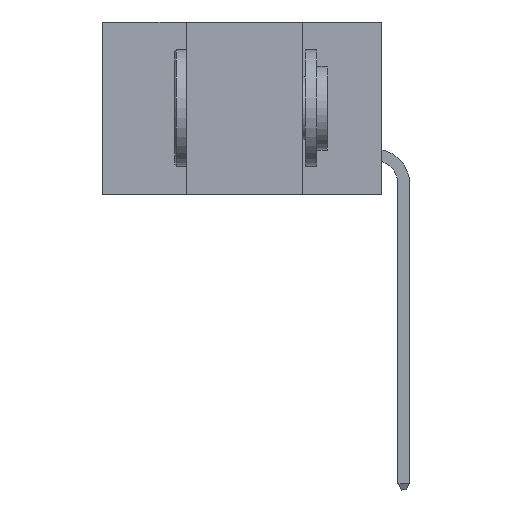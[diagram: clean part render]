
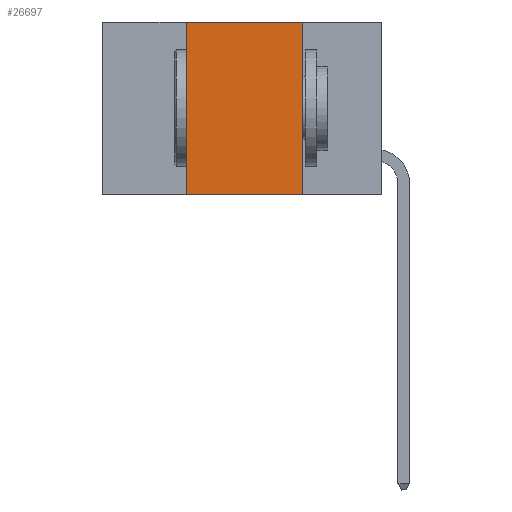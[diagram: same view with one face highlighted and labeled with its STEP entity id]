
A CAD part, left-side view. The second image highlights one B-rep face of the part: STEP entity #26697.
In plain terms, the highlighted planar face has unit normal (-1, 0, 0).
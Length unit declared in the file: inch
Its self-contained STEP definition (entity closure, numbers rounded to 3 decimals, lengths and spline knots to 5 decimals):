
#749 = ORIENTED_EDGE ( 'NONE', *, *, #1945, .F. ) ;
#993 = VERTEX_POINT ( 'NONE', #15844 ) ;
#1127 = CARTESIAN_POINT ( 'NONE',  ( 0., 0.17, 0. ) ) ;
#1232 = VECTOR ( 'NONE', #5540, 39.37008 ) ;
#1625 = EDGE_CURVE ( 'NONE', #14627, #6044, #10983, .T. ) ;
#1945 = EDGE_CURVE ( 'NONE', #6044, #993, #24917, .T. ) ;
#3976 = DIRECTION ( 'NONE',  ( 0., -1., 0. ) ) ;
#5540 = DIRECTION ( 'NONE',  ( 0., 0., -1. ) ) ;
#5875 = VECTOR ( 'NONE', #21175, 39.37008 ) ;
#6044 = VERTEX_POINT ( 'NONE', #8554 ) ;
#6115 = CARTESIAN_POINT ( 'NONE',  ( 0., 0.6, 0. ) ) ;
#6715 = EDGE_LOOP ( 'NONE', ( #18920, #749, #20619, #13876 ) ) ;
#7058 = LINE ( 'NONE', #1127, #1232 ) ;
#7191 = CARTESIAN_POINT ( 'NONE',  ( 0., 0.42, -0.37 ) ) ;
#8554 = CARTESIAN_POINT ( 'NONE',  ( 0., 0.42, 0. ) ) ;
#9179 = AXIS2_PLACEMENT_3D ( 'NONE', #6115, #25692, #12681 ) ;
#10320 = CARTESIAN_POINT ( 'NONE',  ( 0., 0.42, 0. ) ) ;
#10983 = LINE ( 'NONE', #10320, #5875 ) ;
#12681 = DIRECTION ( 'NONE',  ( 0., 0., -1. ) ) ;
#13876 = ORIENTED_EDGE ( 'NONE', *, *, #15181, .T. ) ;
#14627 = VERTEX_POINT ( 'NONE', #7191 ) ;
#15181 = EDGE_CURVE ( 'NONE', #14627, #27091, #23804, .T. ) ;
#15844 = CARTESIAN_POINT ( 'NONE',  ( 0., 0.17, 0. ) ) ;
#16355 = CARTESIAN_POINT ( 'NONE',  ( 0., 0.6, 0. ) ) ;
#16989 = FACE_OUTER_BOUND ( 'NONE', #6715, .T. ) ;
#17029 = VECTOR ( 'NONE', #24287, 39.37008 ) ;
#18128 = CARTESIAN_POINT ( 'NONE',  ( 0., 0.17, -0.37 ) ) ;
#18920 = ORIENTED_EDGE ( 'NONE', *, *, #28053, .F. ) ;
#19149 = PLANE ( 'NONE',  #9179 ) ;
#20619 = ORIENTED_EDGE ( 'NONE', *, *, #1625, .F. ) ;
#21175 = DIRECTION ( 'NONE',  ( 0., 0., 1. ) ) ;
#21878 = VECTOR ( 'NONE', #3976, 39.37008 ) ;
#23804 = LINE ( 'NONE', #26561, #17029 ) ;
#24287 = DIRECTION ( 'NONE',  ( 0., -1., 0. ) ) ;
#24917 = LINE ( 'NONE', #16355, #21878 ) ;
#25692 = DIRECTION ( 'NONE',  ( 1., 0., 0. ) ) ;
#26561 = CARTESIAN_POINT ( 'NONE',  ( 0., 0.6, -0.37 ) ) ;
#26697 = ADVANCED_FACE ( 'NONE', ( #16989 ), #19149, .F. ) ;
#27091 = VERTEX_POINT ( 'NONE', #18128 ) ;
#28053 = EDGE_CURVE ( 'NONE', #993, #27091, #7058, .T. ) ;
